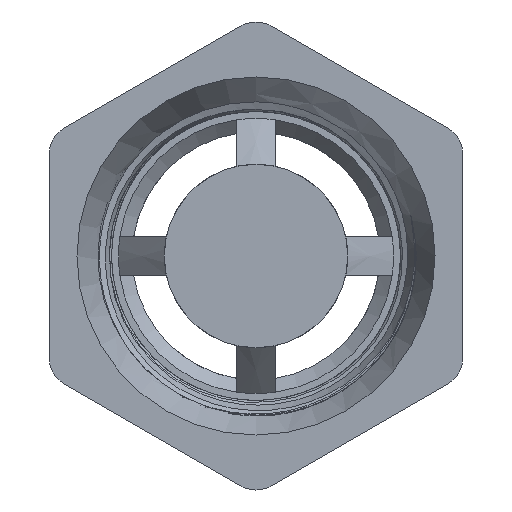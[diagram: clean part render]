
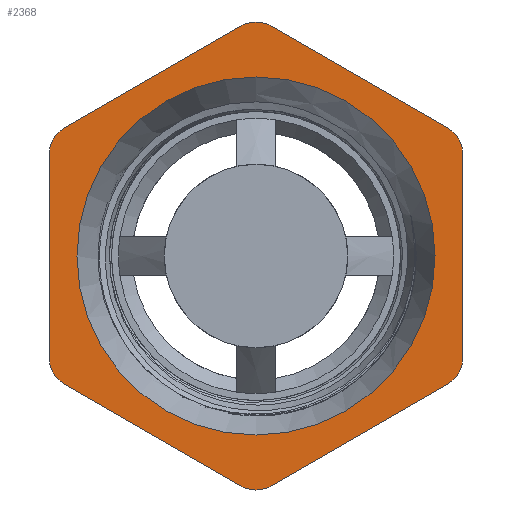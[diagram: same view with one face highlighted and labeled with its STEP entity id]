
A CAD part, front view. The second image highlights one B-rep face of the part: STEP entity #2368.
In plain terms, the highlighted planar face has unit normal (0, -1, 0).
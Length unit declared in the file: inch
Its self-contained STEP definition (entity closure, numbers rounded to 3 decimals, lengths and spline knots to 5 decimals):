
#23=FACE_BOUND('',#363,.T.);
#83=PLANE('',#2615);
#233=FACE_OUTER_BOUND('',#362,.T.);
#362=EDGE_LOOP('',(#2138,#2139,#2140,#2141,#2142,#2143,#2144,#2145,#2146,
#2147,#2148,#2149));
#363=EDGE_LOOP('',(#2150,#2151));
#374=CIRCLE('',#2412,0.46109);
#375=CIRCLE('',#2413,0.46109);
#468=CIRCLE('',#2592,0.07874);
#473=CIRCLE('',#2602,0.07874);
#474=CIRCLE('',#2604,0.07874);
#475=CIRCLE('',#2606,0.07874);
#476=CIRCLE('',#2608,0.07874);
#477=CIRCLE('',#2610,0.07874);
#698=LINE('',#10373,#827);
#714=LINE('',#10495,#843);
#715=LINE('',#10497,#844);
#718=LINE('',#13270,#847);
#719=LINE('',#13271,#848);
#720=LINE('',#13272,#849);
#827=VECTOR('',#3076,0.3937);
#843=VECTOR('',#3180,0.3937);
#844=VECTOR('',#3183,0.3937);
#847=VECTOR('',#3192,0.3937);
#848=VECTOR('',#3193,0.3937);
#849=VECTOR('',#3194,0.3937);
#903=VERTEX_POINT('',#3908);
#904=VERTEX_POINT('',#3909);
#1071=VERTEX_POINT('',#10370);
#1072=VERTEX_POINT('',#10372);
#1079=VERTEX_POINT('',#10455);
#1080=VERTEX_POINT('',#10467);
#1081=VERTEX_POINT('',#10469);
#1082=VERTEX_POINT('',#10473);
#1083=VERTEX_POINT('',#10475);
#1084=VERTEX_POINT('',#10479);
#1085=VERTEX_POINT('',#10481);
#1086=VERTEX_POINT('',#10485);
#1087=VERTEX_POINT('',#10487);
#1088=VERTEX_POINT('',#10491);
#1154=EDGE_CURVE('',#903,#904,#374,.T.);
#1155=EDGE_CURVE('',#904,#903,#375,.T.);
#1407=EDGE_CURVE('',#1072,#1071,#698,.T.);
#1427=EDGE_CURVE('',#1072,#1079,#468,.T.);
#1434=EDGE_CURVE('',#1080,#1081,#473,.T.);
#1437=EDGE_CURVE('',#1082,#1083,#474,.T.);
#1440=EDGE_CURVE('',#1084,#1085,#475,.T.);
#1444=EDGE_CURVE('',#1087,#1086,#476,.T.);
#1445=EDGE_CURVE('',#1088,#1071,#477,.T.);
#1447=EDGE_CURVE('',#1080,#1085,#714,.T.);
#1448=EDGE_CURVE('',#1084,#1079,#715,.T.);
#1455=EDGE_CURVE('',#1088,#1086,#718,.T.);
#1456=EDGE_CURVE('',#1087,#1083,#719,.T.);
#1457=EDGE_CURVE('',#1082,#1081,#720,.T.);
#2138=ORIENTED_EDGE('',*,*,#1434,.F.);
#2139=ORIENTED_EDGE('',*,*,#1447,.T.);
#2140=ORIENTED_EDGE('',*,*,#1440,.F.);
#2141=ORIENTED_EDGE('',*,*,#1448,.T.);
#2142=ORIENTED_EDGE('',*,*,#1427,.F.);
#2143=ORIENTED_EDGE('',*,*,#1407,.T.);
#2144=ORIENTED_EDGE('',*,*,#1445,.F.);
#2145=ORIENTED_EDGE('',*,*,#1455,.T.);
#2146=ORIENTED_EDGE('',*,*,#1444,.F.);
#2147=ORIENTED_EDGE('',*,*,#1456,.T.);
#2148=ORIENTED_EDGE('',*,*,#1437,.F.);
#2149=ORIENTED_EDGE('',*,*,#1457,.T.);
#2150=ORIENTED_EDGE('',*,*,#1154,.T.);
#2151=ORIENTED_EDGE('',*,*,#1155,.T.);
#2368=ADVANCED_FACE('',(#233,#23),#83,.T.);
#2412=AXIS2_PLACEMENT_3D('',#3910,#2671,#2672);
#2413=AXIS2_PLACEMENT_3D('',#3911,#2673,#2674);
#2592=AXIS2_PLACEMENT_3D('',#10456,#3130,#3131);
#2602=AXIS2_PLACEMENT_3D('',#10470,#3152,#3153);
#2604=AXIS2_PLACEMENT_3D('',#10476,#3158,#3159);
#2606=AXIS2_PLACEMENT_3D('',#10482,#3164,#3165);
#2608=AXIS2_PLACEMENT_3D('',#10489,#3171,#3172);
#2610=AXIS2_PLACEMENT_3D('',#10492,#3175,#3176);
#2615=AXIS2_PLACEMENT_3D('',#13269,#3190,#3191);
#2671=DIRECTION('center_axis',(0.,1.,0.));
#2672=DIRECTION('ref_axis',(0.,0.,-1.));
#2673=DIRECTION('center_axis',(0.,1.,0.));
#2674=DIRECTION('ref_axis',(0.,0.,-1.));
#3076=DIRECTION('',(0.,0.,1.));
#3130=DIRECTION('center_axis',(0.,1.,0.));
#3131=DIRECTION('ref_axis',(0.866,0.,-0.5));
#3152=DIRECTION('center_axis',(0.,1.,0.));
#3153=DIRECTION('ref_axis',(-0.866,0.,-0.5));
#3158=DIRECTION('center_axis',(0.,1.,0.));
#3159=DIRECTION('ref_axis',(-0.866,0.,0.5));
#3164=DIRECTION('center_axis',(0.,1.,0.));
#3165=DIRECTION('ref_axis',(0.,0.,-1.));
#3171=DIRECTION('center_axis',(0.,1.,0.));
#3172=DIRECTION('ref_axis',(0.,0.,1.));
#3175=DIRECTION('center_axis',(0.,1.,0.));
#3176=DIRECTION('ref_axis',(0.866,0.,0.5));
#3180=DIRECTION('',(0.866,0.,-0.5));
#3183=DIRECTION('',(0.866,0.,0.5));
#3190=DIRECTION('center_axis',(0.,-1.,0.));
#3191=DIRECTION('ref_axis',(0.,0.,-1.));
#3192=DIRECTION('',(-0.866,0.,0.5));
#3193=DIRECTION('',(-0.866,0.,-0.5));
#3194=DIRECTION('',(0.,0.,-1.));
#3908=CARTESIAN_POINT('',(0.,-1.,-0.46109));
#3909=CARTESIAN_POINT('',(0.,-1.,0.46109));
#3910=CARTESIAN_POINT('Origin',(0.,-1.,0.));
#3911=CARTESIAN_POINT('Origin',(0.,-1.,0.));
#10370=CARTESIAN_POINT('',(0.53242,-1.,0.26193));
#10372=CARTESIAN_POINT('',(0.53242,-1.,-0.26193));
#10373=CARTESIAN_POINT('',(0.53242,-1.,-0.30739));
#10455=CARTESIAN_POINT('',(0.49305,-1.,-0.33012));
#10456=CARTESIAN_POINT('Origin',(0.45368,-1.,-0.26193));
#10467=CARTESIAN_POINT('',(-0.49305,-1.,-0.33012));
#10469=CARTESIAN_POINT('',(-0.53242,-1.,-0.26193));
#10470=CARTESIAN_POINT('Origin',(-0.45368,-1.,-0.26193));
#10473=CARTESIAN_POINT('',(-0.53242,-1.,0.26193));
#10475=CARTESIAN_POINT('',(-0.49305,-1.,0.33012));
#10476=CARTESIAN_POINT('Origin',(-0.45368,-1.,0.26193));
#10479=CARTESIAN_POINT('',(0.03937,-1.,-0.59206));
#10481=CARTESIAN_POINT('',(-0.03937,-1.,-0.59206));
#10482=CARTESIAN_POINT('Origin',(0.,-1.,-0.52387));
#10485=CARTESIAN_POINT('',(0.03937,-1.,0.59206));
#10487=CARTESIAN_POINT('',(-0.03937,-1.,0.59206));
#10489=CARTESIAN_POINT('Origin',(0.,-1.,0.52387));
#10491=CARTESIAN_POINT('',(0.49305,-1.,0.33012));
#10492=CARTESIAN_POINT('Origin',(0.45368,-1.,0.26193));
#10495=CARTESIAN_POINT('',(-0.53242,-1.,-0.30739));
#10497=CARTESIAN_POINT('',(0.,-1.,-0.61479));
#13269=CARTESIAN_POINT('Origin',(0.,-1.,0.));
#13270=CARTESIAN_POINT('',(0.53242,-1.,0.30739));
#13271=CARTESIAN_POINT('',(0.,-1.,0.61479));
#13272=CARTESIAN_POINT('',(-0.53242,-1.,0.30739));
